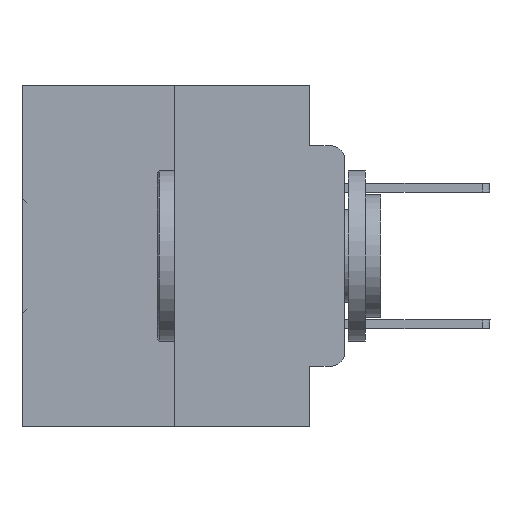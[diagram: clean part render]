
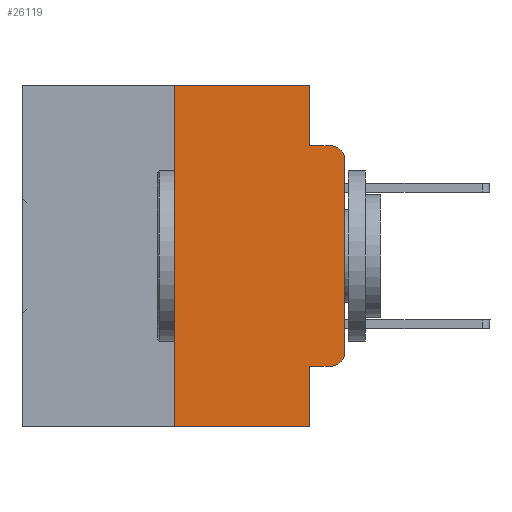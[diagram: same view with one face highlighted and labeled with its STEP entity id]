
A CAD part, left-side view. The second image highlights one B-rep face of the part: STEP entity #26119.
In plain terms, the highlighted planar face has unit normal (-1, 0, 0).
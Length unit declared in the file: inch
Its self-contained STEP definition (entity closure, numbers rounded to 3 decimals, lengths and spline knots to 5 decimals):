
#771 = VERTEX_POINT ( 'NONE', #23306 ) ;
#862 = EDGE_CURVE ( 'NONE', #26440, #12146, #30245, .T. ) ;
#1480 = CARTESIAN_POINT ( 'NONE',  ( 0., 0.051, 0. ) ) ;
#1705 = LINE ( 'NONE', #31224, #10712 ) ;
#1739 = VERTEX_POINT ( 'NONE', #31574 ) ;
#1740 = DIRECTION ( 'NONE',  ( 0., -1., 0. ) ) ;
#2512 = AXIS2_PLACEMENT_3D ( 'NONE', #24869, #11424, #30714 ) ;
#3974 = EDGE_LOOP ( 'NONE', ( #34680, #10412, #16004, #22229, #18639, #19407, #10563, #28561, #17010, #13604 ) ) ;
#4082 = EDGE_CURVE ( 'NONE', #14695, #12146, #12099, .T. ) ;
#4587 = CARTESIAN_POINT ( 'NONE',  ( 0., 0., 0. ) ) ;
#4844 = CARTESIAN_POINT ( 'NONE',  ( 0., 0.02, -0.1085 ) ) ;
#5370 = CARTESIAN_POINT ( 'NONE',  ( 0., 0.051, -0.0885 ) ) ;
#5606 = VECTOR ( 'NONE', #26555, 39.37008 ) ;
#6983 = FACE_OUTER_BOUND ( 'NONE', #3974, .T. ) ;
#8187 = DIRECTION ( 'NONE',  ( 0., -1., 0. ) ) ;
#8697 = DIRECTION ( 'NONE',  ( 0., -1., 0. ) ) ;
#9322 = VECTOR ( 'NONE', #8187, 39.37008 ) ;
#9774 = LINE ( 'NONE', #16310, #9322 ) ;
#10412 = ORIENTED_EDGE ( 'NONE', *, *, #862, .T. ) ;
#10563 = ORIENTED_EDGE ( 'NONE', *, *, #16474, .T. ) ;
#10634 = EDGE_CURVE ( 'NONE', #25108, #26440, #34623, .T. ) ;
#10712 = VECTOR ( 'NONE', #1740, 39.37008 ) ;
#10893 = DIRECTION ( 'NONE',  ( 0., -1., 0. ) ) ;
#11348 = CARTESIAN_POINT ( 'NONE',  ( 0., 0.25, 0. ) ) ;
#11424 = DIRECTION ( 'NONE',  ( -1., 0., 0. ) ) ;
#12099 = LINE ( 'NONE', #5370, #24009 ) ;
#12146 = VERTEX_POINT ( 'NONE', #20613 ) ;
#12351 = CARTESIAN_POINT ( 'NONE',  ( 0., 0.25, 0. ) ) ;
#12953 = CARTESIAN_POINT ( 'NONE',  ( 0., 0.051, -0.5 ) ) ;
#13213 = EDGE_CURVE ( 'NONE', #771, #14695, #30419, .T. ) ;
#13604 = ORIENTED_EDGE ( 'NONE', *, *, #22002, .T. ) ;
#13739 = LINE ( 'NONE', #14856, #18425 ) ;
#13968 = EDGE_CURVE ( 'NONE', #34004, #33951, #13739, .T. ) ;
#14695 = VERTEX_POINT ( 'NONE', #23167 ) ;
#14856 = CARTESIAN_POINT ( 'NONE',  ( 0., 0.051, 0. ) ) ;
#15769 = AXIS2_PLACEMENT_3D ( 'NONE', #31368, #17418, #28616 ) ;
#16004 = ORIENTED_EDGE ( 'NONE', *, *, #4082, .F. ) ;
#16310 = CARTESIAN_POINT ( 'NONE',  ( 0., 0.473, 0. ) ) ;
#16474 = EDGE_CURVE ( 'NONE', #1739, #33951, #32782, .T. ) ;
#16754 = VERTEX_POINT ( 'NONE', #12351 ) ;
#17010 = ORIENTED_EDGE ( 'NONE', *, *, #33839, .T. ) ;
#17418 = DIRECTION ( 'NONE',  ( 1., 0., 0. ) ) ;
#18064 = AXIS2_PLACEMENT_3D ( 'NONE', #4844, #21444, #29305 ) ;
#18425 = VECTOR ( 'NONE', #28552, 39.37008 ) ;
#18639 = ORIENTED_EDGE ( 'NONE', *, *, #29707, .F. ) ;
#19407 = ORIENTED_EDGE ( 'NONE', *, *, #27802, .F. ) ;
#19916 = CARTESIAN_POINT ( 'NONE',  ( 0., 0.473, -0.5 ) ) ;
#20401 = PLANE ( 'NONE',  #15769 ) ;
#20585 = DIRECTION ( 'NONE',  ( 0., 0., -1. ) ) ;
#20613 = CARTESIAN_POINT ( 'NONE',  ( 0., 0.02, -0.0885 ) ) ;
#21332 = CARTESIAN_POINT ( 'NONE',  ( 0., 0., -0.1085 ) ) ;
#21444 = DIRECTION ( 'NONE',  ( -1., 0., 0. ) ) ;
#22002 = EDGE_CURVE ( 'NONE', #29512, #25108, #30645, .T. ) ;
#22229 = ORIENTED_EDGE ( 'NONE', *, *, #13213, .F. ) ;
#23165 = VECTOR ( 'NONE', #20585, 39.37008 ) ;
#23167 = CARTESIAN_POINT ( 'NONE',  ( 0., 0.051, -0.0885 ) ) ;
#23306 = CARTESIAN_POINT ( 'NONE',  ( 0., 0.051, 0. ) ) ;
#24009 = VECTOR ( 'NONE', #10893, 39.37008 ) ;
#24869 = CARTESIAN_POINT ( 'NONE',  ( 0., 0.02, -0.3915 ) ) ;
#24908 = DIRECTION ( 'NONE',  ( 0., 0., 1. ) ) ;
#25108 = VERTEX_POINT ( 'NONE', #32721 ) ;
#25243 = VECTOR ( 'NONE', #24908, 39.37008 ) ;
#26119 = ADVANCED_FACE ( 'NONE', ( #6983 ), #20401, .F. ) ;
#26440 = VERTEX_POINT ( 'NONE', #21332 ) ;
#26555 = DIRECTION ( 'NONE',  ( 0., 0., 1. ) ) ;
#27802 = EDGE_CURVE ( 'NONE', #1739, #16754, #32498, .T. ) ;
#28552 = DIRECTION ( 'NONE',  ( 0., 0., -1. ) ) ;
#28561 = ORIENTED_EDGE ( 'NONE', *, *, #13968, .F. ) ;
#28616 = DIRECTION ( 'NONE',  ( 0., 0., -1. ) ) ;
#29305 = DIRECTION ( 'NONE',  ( 0., 0., -1. ) ) ;
#29512 = VERTEX_POINT ( 'NONE', #31699 ) ;
#29707 = EDGE_CURVE ( 'NONE', #16754, #771, #9774, .T. ) ;
#29747 = CARTESIAN_POINT ( 'NONE',  ( 0., 0.051, -0.4115 ) ) ;
#30245 = CIRCLE ( 'NONE', #18064, 0.02 ) ;
#30419 = LINE ( 'NONE', #1480, #23165 ) ;
#30645 = CIRCLE ( 'NONE', #2512, 0.02 ) ;
#30714 = DIRECTION ( 'NONE',  ( 0., 0., -1. ) ) ;
#31224 = CARTESIAN_POINT ( 'NONE',  ( 0., 0.051, -0.4115 ) ) ;
#31368 = CARTESIAN_POINT ( 'NONE',  ( 0., 0.473, 0. ) ) ;
#31574 = CARTESIAN_POINT ( 'NONE',  ( 0., 0.25, -0.5 ) ) ;
#31699 = CARTESIAN_POINT ( 'NONE',  ( 0., 0.02, -0.4115 ) ) ;
#32498 = LINE ( 'NONE', #11348, #25243 ) ;
#32721 = CARTESIAN_POINT ( 'NONE',  ( 0., 0., -0.3915 ) ) ;
#32782 = LINE ( 'NONE', #19916, #34485 ) ;
#33839 = EDGE_CURVE ( 'NONE', #34004, #29512, #1705, .T. ) ;
#33951 = VERTEX_POINT ( 'NONE', #12953 ) ;
#34004 = VERTEX_POINT ( 'NONE', #29747 ) ;
#34485 = VECTOR ( 'NONE', #8697, 39.37008 ) ;
#34623 = LINE ( 'NONE', #4587, #5606 ) ;
#34680 = ORIENTED_EDGE ( 'NONE', *, *, #10634, .T. ) ;
